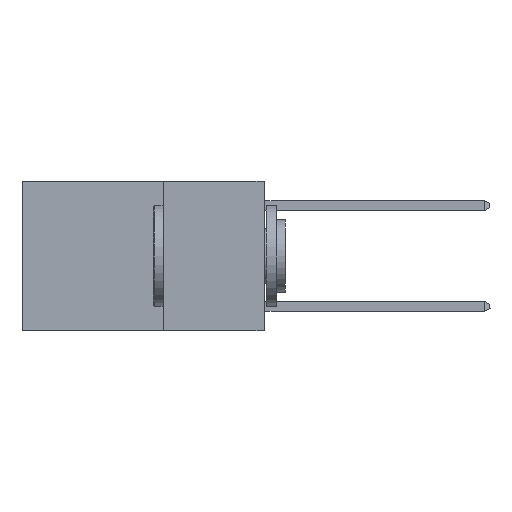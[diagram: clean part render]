
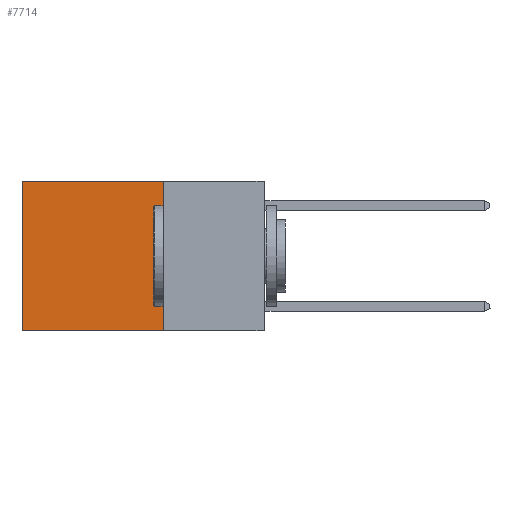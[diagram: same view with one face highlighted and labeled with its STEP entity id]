
A CAD part, left-side view. The second image highlights one B-rep face of the part: STEP entity #7714.
In plain terms, the highlighted planar face has unit normal (-1, 0, 0).
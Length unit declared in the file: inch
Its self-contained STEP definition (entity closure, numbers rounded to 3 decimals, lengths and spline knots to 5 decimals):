
#1308 = CARTESIAN_POINT ( 'NONE',  ( 0.2625, 0.25, 0. ) ) ;
#1676 = ORIENTED_EDGE ( 'NONE', *, *, #14288, .T. ) ;
#3320 = EDGE_LOOP ( 'NONE', ( #1676, #27724, #25569, #6568 ) ) ;
#3557 = DIRECTION ( 'NONE',  ( 0., 0., -1. ) ) ;
#5248 = CARTESIAN_POINT ( 'NONE',  ( 0.2625, 0.25, 0. ) ) ;
#6568 = ORIENTED_EDGE ( 'NONE', *, *, #12334, .T. ) ;
#7186 = CARTESIAN_POINT ( 'NONE',  ( 0.2625, 0.6, 0. ) ) ;
#7429 = DIRECTION ( 'NONE',  ( 0., 1., 0. ) ) ;
#7714 = ADVANCED_FACE ( 'NONE', ( #24902 ), #20325, .F. ) ;
#7821 = VERTEX_POINT ( 'NONE', #12090 ) ;
#8310 = EDGE_CURVE ( 'NONE', #24124, #7821, #17093, .T. ) ;
#8654 = CARTESIAN_POINT ( 'NONE',  ( 0.2625, 0.6, 0. ) ) ;
#8953 = VECTOR ( 'NONE', #3557, 39.37008 ) ;
#9641 = DIRECTION ( 'NONE',  ( 0., 0., -1. ) ) ;
#10303 = EDGE_CURVE ( 'NONE', #27013, #24124, #24089, .T. ) ;
#10366 = CARTESIAN_POINT ( 'NONE',  ( 0.2625, 0.25, 0. ) ) ;
#11383 = VECTOR ( 'NONE', #27195, 39.37008 ) ;
#11704 = CARTESIAN_POINT ( 'NONE',  ( 0.2625, 0.25, 0. ) ) ;
#12090 = CARTESIAN_POINT ( 'NONE',  ( 0.2625, 0.6, -0.37 ) ) ;
#12334 = EDGE_CURVE ( 'NONE', #27013, #19137, #19243, .T. ) ;
#13015 = DIRECTION ( 'NONE',  ( 0., 0., -1. ) ) ;
#13585 = VECTOR ( 'NONE', #7429, 39.37008 ) ;
#14194 = LINE ( 'NONE', #8654, #19173 ) ;
#14288 = EDGE_CURVE ( 'NONE', #19137, #7821, #14194, .T. ) ;
#15938 = CARTESIAN_POINT ( 'NONE',  ( 0.2625, 0.25, -0.37 ) ) ;
#17093 = LINE ( 'NONE', #25000, #11383 ) ;
#19137 = VERTEX_POINT ( 'NONE', #7186 ) ;
#19173 = VECTOR ( 'NONE', #13015, 39.37008 ) ;
#19243 = LINE ( 'NONE', #11704, #13585 ) ;
#20325 = PLANE ( 'NONE',  #27090 ) ;
#22503 = DIRECTION ( 'NONE',  ( 1., 0., 0. ) ) ;
#24089 = LINE ( 'NONE', #1308, #8953 ) ;
#24124 = VERTEX_POINT ( 'NONE', #15938 ) ;
#24902 = FACE_OUTER_BOUND ( 'NONE', #3320, .T. ) ;
#25000 = CARTESIAN_POINT ( 'NONE',  ( 0.2625, 0.25, -0.37 ) ) ;
#25569 = ORIENTED_EDGE ( 'NONE', *, *, #10303, .F. ) ;
#27013 = VERTEX_POINT ( 'NONE', #10366 ) ;
#27090 = AXIS2_PLACEMENT_3D ( 'NONE', #5248, #22503, #9641 ) ;
#27195 = DIRECTION ( 'NONE',  ( 0., 1., 0. ) ) ;
#27724 = ORIENTED_EDGE ( 'NONE', *, *, #8310, .F. ) ;
